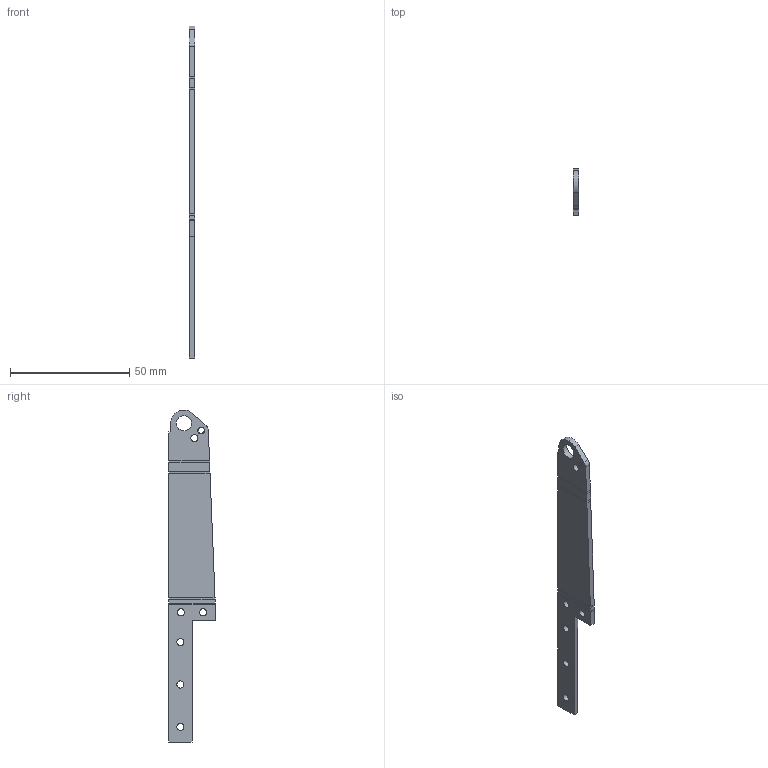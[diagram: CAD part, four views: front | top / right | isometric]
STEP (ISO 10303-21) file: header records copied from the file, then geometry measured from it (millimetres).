
FILE_DESCRIPTION(/* description */ (''),/* implementation_level */ '2;1');
FILE_NAME(/* name */ 'Front SR Side Plate 47 Flat.step',/* time_stamp */ '2024-01-16T16:19:37-05:00',/* author */ (''),/* organization */ (''),/* preprocessor_version */ 'ST-DEVELOPER v20',/* originating_system */ 'Autodesk Translation Framework v12.14.0.127',/* authorisation */ '');
FILE_SCHEMA (('AUTOMOTIVE_DESIGN { 1 0 10303 214 3 1 1 }'));
Length unit declared in the file: inch
Products named in the file (1): AR47 Magwell
Bounding box: 2.29 x 19.51 x 139.32 mm (x, y, z)
Volume: 4496.4 mm3; surface area: 4845.3 mm2
Topology: 1 solids, 1 shells, 66 faces, 159 edges, 95 vertices
Faces by surface type: plane 40, cylinder 20, bspline 6
Full cylindrical faces by diameter (mm): 2.529 x1, 3 x6, 3.086 x1, 6.426 x1
Entity records: 2662 total; most frequent: CARTESIAN_POINT 1145, ORIENTED_EDGE 318, DIRECTION 269, EDGE_CURVE 159, LINE 103, VECTOR 103, VERTEX_POINT 95, AXIS2_PLACEMENT_3D 83
